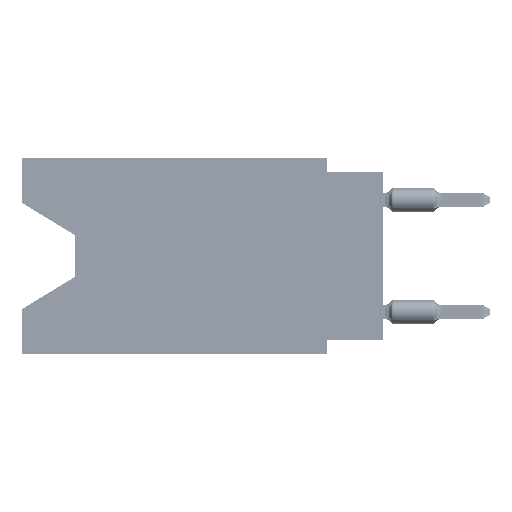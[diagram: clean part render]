
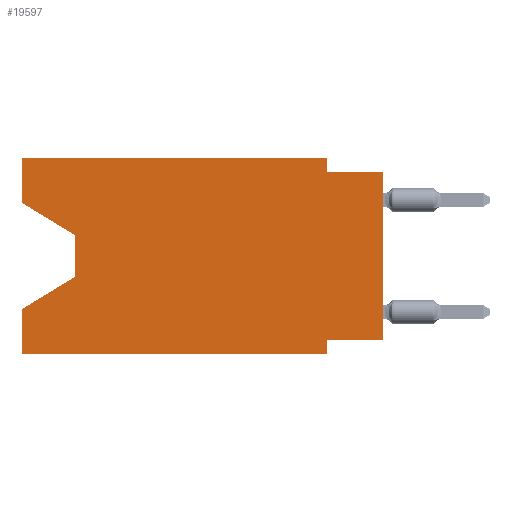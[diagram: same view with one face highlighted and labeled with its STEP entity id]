
A CAD part, left-side view. The second image highlights one B-rep face of the part: STEP entity #19597.
In plain terms, the highlighted planar face has unit normal (-1, 0, 0).
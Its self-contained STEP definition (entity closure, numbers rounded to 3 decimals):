
#1296 = PLANE ( 'NONE',  #22952 ) ;
#1335 = VECTOR ( 'NONE', #59532, 1000. ) ;
#1352 = EDGE_CURVE ( 'NONE', #67720, #28789, #11093, .T. ) ;
#2305 = ORIENTED_EDGE ( 'NONE', *, *, #23549, .T. ) ;
#2591 = EDGE_LOOP ( 'NONE', ( #91733, #22978, #104712, #20671, #10646, #43649, #53215, #2305, #94601, #94256, #17311, #68138 ) ) ;
#2624 = CARTESIAN_POINT ( 'NONE',  ( 0., 2.54, 0. ) ) ;
#2680 = EDGE_CURVE ( 'NONE', #37202, #41574, #99140, .T. ) ;
#3435 = DIRECTION ( 'NONE',  ( 0., 0., -1. ) ) ;
#5099 = EDGE_CURVE ( 'NONE', #97264, #105324, #96651, .T. ) ;
#5254 = DIRECTION ( 'NONE',  ( 0., 1., 0. ) ) ;
#5805 = CARTESIAN_POINT ( 'NONE',  ( 0., 16.383, -2.038 ) ) ;
#7937 = LINE ( 'NONE', #90723, #103267 ) ;
#10413 = CARTESIAN_POINT ( 'NONE',  ( 0., 16.383, 0. ) ) ;
#10492 = VERTEX_POINT ( 'NONE', #53103 ) ;
#10646 = ORIENTED_EDGE ( 'NONE', *, *, #64581, .T. ) ;
#10734 = VECTOR ( 'NONE', #3435, 1000. ) ;
#11093 = LINE ( 'NONE', #99856, #1335 ) ;
#12154 = EDGE_CURVE ( 'NONE', #28789, #48849, #14310, .T. ) ;
#14310 = LINE ( 'NONE', #80993, #92516 ) ;
#16181 = VERTEX_POINT ( 'NONE', #72242 ) ;
#17311 = ORIENTED_EDGE ( 'NONE', *, *, #104397, .F. ) ;
#18484 = EDGE_CURVE ( 'NONE', #99673, #16181, #28692, .T. ) ;
#19597 = ADVANCED_FACE ( 'NONE', ( #74978 ), #1296, .F. ) ;
#20671 = ORIENTED_EDGE ( 'NONE', *, *, #33317, .F. ) ;
#21167 = CARTESIAN_POINT ( 'NONE',  ( 0., 2.54, 0. ) ) ;
#21802 = CARTESIAN_POINT ( 'NONE',  ( 0., 13.97, -3.505 ) ) ;
#22952 = AXIS2_PLACEMENT_3D ( 'NONE', #57282, #65869, #24454 ) ;
#22978 = ORIENTED_EDGE ( 'NONE', *, *, #1352, .T. ) ;
#23087 = LINE ( 'NONE', #89745, #24571 ) ;
#23549 = EDGE_CURVE ( 'NONE', #97264, #70930, #92260, .T. ) ;
#24454 = DIRECTION ( 'NONE',  ( 0., 0., -1. ) ) ;
#24571 = VECTOR ( 'NONE', #30612, 1000. ) ;
#27031 = CARTESIAN_POINT ( 'NONE',  ( 0., 16.383, 0. ) ) ;
#27172 = DIRECTION ( 'NONE',  ( 0., 0., 1. ) ) ;
#28692 = LINE ( 'NONE', #21167, #10734 ) ;
#28789 = VERTEX_POINT ( 'NONE', #60259 ) ;
#28826 = CARTESIAN_POINT ( 'NONE',  ( 0., 16.383, -8.89 ) ) ;
#29971 = CARTESIAN_POINT ( 'NONE',  ( 0., 0., -8.255 ) ) ;
#30612 = DIRECTION ( 'NONE',  ( 0., 0., 1. ) ) ;
#32660 = DIRECTION ( 'NONE',  ( 0., -0.855, -0.519 ) ) ;
#33317 = EDGE_CURVE ( 'NONE', #104594, #48849, #23087, .T. ) ;
#36297 = LINE ( 'NONE', #101371, #41306 ) ;
#36582 = CARTESIAN_POINT ( 'NONE',  ( 0., 16.383, 0. ) ) ;
#36826 = DIRECTION ( 'NONE',  ( 0., -1., 0. ) ) ;
#37202 = VERTEX_POINT ( 'NONE', #5805 ) ;
#38016 = CARTESIAN_POINT ( 'NONE',  ( 0., 16.383, -6.852 ) ) ;
#41306 = VECTOR ( 'NONE', #36826, 1000. ) ;
#41320 = CARTESIAN_POINT ( 'NONE',  ( 0., 0., -8.255 ) ) ;
#41574 = VERTEX_POINT ( 'NONE', #10413 ) ;
#43649 = ORIENTED_EDGE ( 'NONE', *, *, #89239, .F. ) ;
#43695 = VECTOR ( 'NONE', #46938, 1000. ) ;
#44657 = LINE ( 'NONE', #36582, #75692 ) ;
#46938 = DIRECTION ( 'NONE',  ( 0., 0., -1. ) ) ;
#48849 = VERTEX_POINT ( 'NONE', #38016 ) ;
#52202 = DIRECTION ( 'NONE',  ( 0., -1., 0. ) ) ;
#53103 = CARTESIAN_POINT ( 'NONE',  ( 0., 2.54, -8.89 ) ) ;
#53215 = ORIENTED_EDGE ( 'NONE', *, *, #5099, .F. ) ;
#54795 = CARTESIAN_POINT ( 'NONE',  ( 0., 0., -0.635 ) ) ;
#57282 = CARTESIAN_POINT ( 'NONE',  ( 0., 16.383, 0. ) ) ;
#58299 = DIRECTION ( 'NONE',  ( 0., 0., 1. ) ) ;
#58323 = VECTOR ( 'NONE', #5254, 1000. ) ;
#59532 = DIRECTION ( 'NONE',  ( 0., 0., -1. ) ) ;
#60259 = CARTESIAN_POINT ( 'NONE',  ( 0., 13.97, -5.385 ) ) ;
#64581 = EDGE_CURVE ( 'NONE', #104594, #10492, #100384, .T. ) ;
#65869 = DIRECTION ( 'NONE',  ( 1., 0., 0. ) ) ;
#67530 = CARTESIAN_POINT ( 'NONE',  ( 0., 0., 0. ) ) ;
#67720 = VERTEX_POINT ( 'NONE', #21802 ) ;
#68138 = ORIENTED_EDGE ( 'NONE', *, *, #2680, .F. ) ;
#69194 = DIRECTION ( 'NONE',  ( 0., -1., 0. ) ) ;
#69553 = CARTESIAN_POINT ( 'NONE',  ( 0., 2.54, -8.255 ) ) ;
#70930 = VERTEX_POINT ( 'NONE', #54795 ) ;
#72242 = CARTESIAN_POINT ( 'NONE',  ( 0., 2.54, -0.635 ) ) ;
#74978 = FACE_OUTER_BOUND ( 'NONE', #2591, .T. ) ;
#75692 = VECTOR ( 'NONE', #52202, 1000. ) ;
#77094 = VECTOR ( 'NONE', #58299, 1000. ) ;
#79065 = CARTESIAN_POINT ( 'NONE',  ( 0., 16.383, -8.89 ) ) ;
#79750 = CARTESIAN_POINT ( 'NONE',  ( 0., 2.54, -8.89 ) ) ;
#80993 = CARTESIAN_POINT ( 'NONE',  ( 0., 13.97, -5.385 ) ) ;
#88513 = DIRECTION ( 'NONE',  ( 0., 0.855, -0.519 ) ) ;
#89239 = EDGE_CURVE ( 'NONE', #105324, #10492, #102348, .T. ) ;
#89745 = CARTESIAN_POINT ( 'NONE',  ( 0., 16.383, 0. ) ) ;
#90723 = CARTESIAN_POINT ( 'NONE',  ( 0., 16.383, -2.038 ) ) ;
#91733 = ORIENTED_EDGE ( 'NONE', *, *, #98367, .T. ) ;
#91876 = VECTOR ( 'NONE', #27172, 1000. ) ;
#92260 = LINE ( 'NONE', #67530, #91876 ) ;
#92516 = VECTOR ( 'NONE', #88513, 1000. ) ;
#94256 = ORIENTED_EDGE ( 'NONE', *, *, #18484, .F. ) ;
#94601 = ORIENTED_EDGE ( 'NONE', *, *, #102329, .F. ) ;
#96651 = LINE ( 'NONE', #29971, #58323 ) ;
#97264 = VERTEX_POINT ( 'NONE', #41320 ) ;
#98367 = EDGE_CURVE ( 'NONE', #37202, #67720, #7937, .T. ) ;
#98915 = VECTOR ( 'NONE', #69194, 1000. ) ;
#99140 = LINE ( 'NONE', #27031, #77094 ) ;
#99673 = VERTEX_POINT ( 'NONE', #2624 ) ;
#99856 = CARTESIAN_POINT ( 'NONE',  ( 0., 13.97, -3.505 ) ) ;
#100384 = LINE ( 'NONE', #28826, #98915 ) ;
#101371 = CARTESIAN_POINT ( 'NONE',  ( 0., 0., -0.635 ) ) ;
#102329 = EDGE_CURVE ( 'NONE', #16181, #70930, #36297, .T. ) ;
#102348 = LINE ( 'NONE', #79750, #43695 ) ;
#103267 = VECTOR ( 'NONE', #32660, 1000. ) ;
#104397 = EDGE_CURVE ( 'NONE', #41574, #99673, #44657, .T. ) ;
#104594 = VERTEX_POINT ( 'NONE', #79065 ) ;
#104712 = ORIENTED_EDGE ( 'NONE', *, *, #12154, .T. ) ;
#105324 = VERTEX_POINT ( 'NONE', #69553 ) ;
